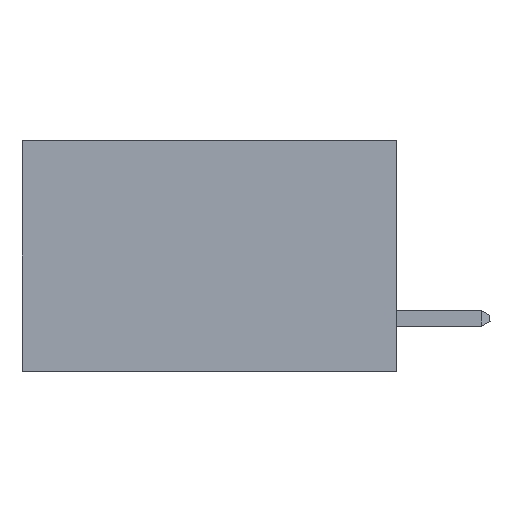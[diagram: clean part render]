
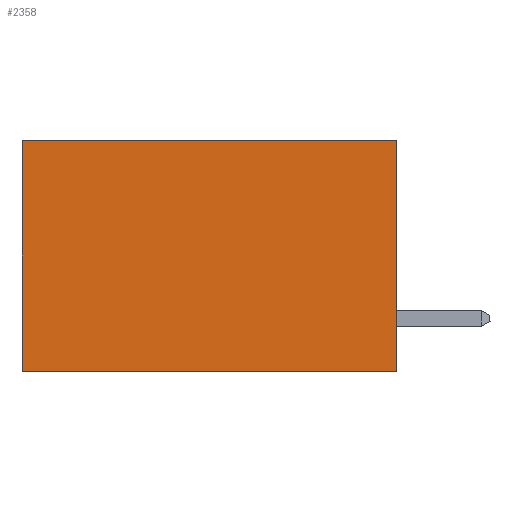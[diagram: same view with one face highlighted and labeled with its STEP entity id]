
A CAD part, left-side view. The second image highlights one B-rep face of the part: STEP entity #2358.
In plain terms, the highlighted planar face has unit normal (-1, 0, 0).
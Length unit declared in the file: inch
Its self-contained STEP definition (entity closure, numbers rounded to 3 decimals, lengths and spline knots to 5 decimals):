
#423 = CARTESIAN_POINT ( 'NONE',  ( 0.298, 0.6, -0.37 ) ) ;
#469 = CARTESIAN_POINT ( 'NONE',  ( 0.298, 0.6, 0. ) ) ;
#886 = CARTESIAN_POINT ( 'NONE',  ( 0.298, 0., 0. ) ) ;
#1606 = DIRECTION ( 'NONE',  ( 0., 0., -1. ) ) ;
#2226 = LINE ( 'NONE', #8260, #9167 ) ;
#2242 = DIRECTION ( 'NONE',  ( 0., 0., -1. ) ) ;
#2358 = ADVANCED_FACE ( 'NONE', ( #12388 ), #17028, .F. ) ;
#2668 = EDGE_CURVE ( 'NONE', #15362, #9871, #10476, .T. ) ;
#2833 = VERTEX_POINT ( 'NONE', #5146 ) ;
#3368 = LINE ( 'NONE', #10238, #13286 ) ;
#4347 = CARTESIAN_POINT ( 'NONE',  ( 0.298, 0.6, 0. ) ) ;
#4690 = EDGE_CURVE ( 'NONE', #15362, #2833, #2226, .T. ) ;
#4895 = AXIS2_PLACEMENT_3D ( 'NONE', #886, #10310, #2242 ) ;
#5146 = CARTESIAN_POINT ( 'NONE',  ( 0.298, 0., -0.37 ) ) ;
#5399 = CARTESIAN_POINT ( 'NONE',  ( 0.298, 0., 0. ) ) ;
#5742 = ORIENTED_EDGE ( 'NONE', *, *, #8205, .F. ) ;
#8205 = EDGE_CURVE ( 'NONE', #2833, #12623, #3368, .T. ) ;
#8260 = CARTESIAN_POINT ( 'NONE',  ( 0.298, 0., 0. ) ) ;
#8632 = EDGE_CURVE ( 'NONE', #9871, #12623, #9286, .T. ) ;
#8978 = ORIENTED_EDGE ( 'NONE', *, *, #2668, .T. ) ;
#9167 = VECTOR ( 'NONE', #9501, 39.37008 ) ;
#9286 = LINE ( 'NONE', #4347, #13470 ) ;
#9501 = DIRECTION ( 'NONE',  ( 0., 0., -1. ) ) ;
#9871 = VERTEX_POINT ( 'NONE', #469 ) ;
#10238 = CARTESIAN_POINT ( 'NONE',  ( 0.298, 0., -0.37 ) ) ;
#10310 = DIRECTION ( 'NONE',  ( 1., 0., 0. ) ) ;
#10476 = LINE ( 'NONE', #15574, #14045 ) ;
#12388 = FACE_OUTER_BOUND ( 'NONE', #12719, .T. ) ;
#12623 = VERTEX_POINT ( 'NONE', #423 ) ;
#12719 = EDGE_LOOP ( 'NONE', ( #17323, #5742, #13088, #8978 ) ) ;
#12933 = DIRECTION ( 'NONE',  ( 0., 1., 0. ) ) ;
#13088 = ORIENTED_EDGE ( 'NONE', *, *, #4690, .F. ) ;
#13286 = VECTOR ( 'NONE', #12933, 39.37008 ) ;
#13470 = VECTOR ( 'NONE', #1606, 39.37008 ) ;
#14045 = VECTOR ( 'NONE', #16918, 39.37008 ) ;
#15362 = VERTEX_POINT ( 'NONE', #5399 ) ;
#15574 = CARTESIAN_POINT ( 'NONE',  ( 0.298, 0., 0. ) ) ;
#16918 = DIRECTION ( 'NONE',  ( 0., 1., 0. ) ) ;
#17028 = PLANE ( 'NONE',  #4895 ) ;
#17323 = ORIENTED_EDGE ( 'NONE', *, *, #8632, .T. ) ;
